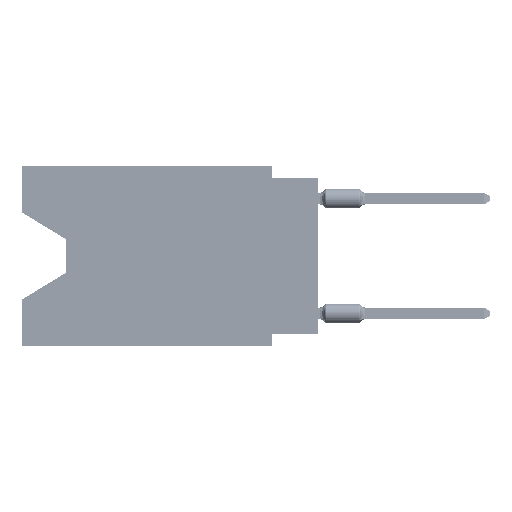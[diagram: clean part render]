
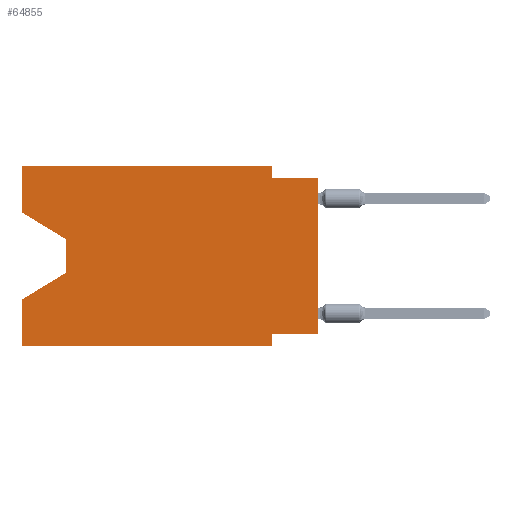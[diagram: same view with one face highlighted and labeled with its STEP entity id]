
A CAD part, left-side view. The second image highlights one B-rep face of the part: STEP entity #64855.
In plain terms, the highlighted planar face has unit normal (-1, 0, 0).
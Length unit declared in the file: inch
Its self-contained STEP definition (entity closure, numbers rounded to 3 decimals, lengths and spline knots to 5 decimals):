
#2189 = DIRECTION ( 'NONE',  ( 0., 0., -1. ) ) ;
#3252 = ORIENTED_EDGE ( 'NONE', *, *, #37040, .F. ) ;
#3545 = VERTEX_POINT ( 'NONE', #38048 ) ;
#3946 = LINE ( 'NONE', #55321, #9532 ) ;
#5629 = CARTESIAN_POINT ( 'NONE',  ( 0., 0.645, 0. ) ) ;
#6065 = ORIENTED_EDGE ( 'NONE', *, *, #27623, .T. ) ;
#6463 = EDGE_CURVE ( 'NONE', #42686, #31544, #49283, .T. ) ;
#7975 = VERTEX_POINT ( 'NONE', #44523 ) ;
#8594 = VERTEX_POINT ( 'NONE', #43351 ) ;
#9532 = VECTOR ( 'NONE', #60090, 39.37008 ) ;
#11187 = DIRECTION ( 'NONE',  ( 0., 0., -1. ) ) ;
#11610 = EDGE_CURVE ( 'NONE', #42686, #52033, #26875, .T. ) ;
#12078 = LINE ( 'NONE', #22346, #57967 ) ;
#12210 = VECTOR ( 'NONE', #60631, 39.37008 ) ;
#12718 = VERTEX_POINT ( 'NONE', #13309 ) ;
#12744 = LINE ( 'NONE', #13426, #60323 ) ;
#13309 = CARTESIAN_POINT ( 'NONE',  ( 0., 0.1, -0.39 ) ) ;
#13426 = CARTESIAN_POINT ( 'NONE',  ( 0., 0., 0. ) ) ;
#14960 = LINE ( 'NONE', #51950, #60369 ) ;
#16079 = ORIENTED_EDGE ( 'NONE', *, *, #6463, .F. ) ;
#16603 = CARTESIAN_POINT ( 'NONE',  ( 0., 0.645, -0.39 ) ) ;
#16934 = VECTOR ( 'NONE', #54395, 39.37008 ) ;
#17810 = CARTESIAN_POINT ( 'NONE',  ( 0., 0.645, -0.10025 ) ) ;
#17923 = FACE_OUTER_BOUND ( 'NONE', #52708, .T. ) ;
#19868 = CARTESIAN_POINT ( 'NONE',  ( 0., 0., -0.025 ) ) ;
#20145 = ORIENTED_EDGE ( 'NONE', *, *, #11610, .T. ) ;
#20229 = ORIENTED_EDGE ( 'NONE', *, *, #62414, .T. ) ;
#20621 = CARTESIAN_POINT ( 'NONE',  ( 0., 0.55, -0.158 ) ) ;
#20980 = CARTESIAN_POINT ( 'NONE',  ( 0., 0.645, -0.39 ) ) ;
#21755 = AXIS2_PLACEMENT_3D ( 'NONE', #59343, #28201, #2189 ) ;
#21877 = EDGE_CURVE ( 'NONE', #61639, #3545, #3946, .T. ) ;
#22346 = CARTESIAN_POINT ( 'NONE',  ( 0., 0.1, 0. ) ) ;
#22469 = VECTOR ( 'NONE', #64134, 39.37008 ) ;
#23143 = CARTESIAN_POINT ( 'NONE',  ( 0., 0.645, -0.28975 ) ) ;
#24936 = EDGE_CURVE ( 'NONE', #52033, #7975, #57927, .T. ) ;
#25849 = DIRECTION ( 'NONE',  ( 0., -0.855, -0.519 ) ) ;
#26875 = LINE ( 'NONE', #31321, #52584 ) ;
#27525 = ORIENTED_EDGE ( 'NONE', *, *, #64669, .F. ) ;
#27623 = EDGE_CURVE ( 'NONE', #7975, #59169, #54735, .T. ) ;
#28201 = DIRECTION ( 'NONE',  ( 1., 0., 0. ) ) ;
#28470 = ORIENTED_EDGE ( 'NONE', *, *, #21877, .F. ) ;
#28643 = ORIENTED_EDGE ( 'NONE', *, *, #33862, .F. ) ;
#29170 = DIRECTION ( 'NONE',  ( 0., 0., 1. ) ) ;
#30195 = EDGE_CURVE ( 'NONE', #53446, #51145, #45559, .T. ) ;
#30322 = VECTOR ( 'NONE', #57950, 39.37008 ) ;
#31321 = CARTESIAN_POINT ( 'NONE',  ( 0., 0.645, -0.10025 ) ) ;
#31506 = CARTESIAN_POINT ( 'NONE',  ( 0., 0., -0.025 ) ) ;
#31544 = VERTEX_POINT ( 'NONE', #57718 ) ;
#33500 = CARTESIAN_POINT ( 'NONE',  ( 0., 0.55, -0.232 ) ) ;
#33862 = EDGE_CURVE ( 'NONE', #3545, #12718, #14960, .T. ) ;
#34720 = CARTESIAN_POINT ( 'NONE',  ( 0., 0.1, -0.025 ) ) ;
#35931 = EDGE_CURVE ( 'NONE', #61639, #51145, #12744, .T. ) ;
#37040 = EDGE_CURVE ( 'NONE', #8594, #53446, #12078, .T. ) ;
#38048 = CARTESIAN_POINT ( 'NONE',  ( 0., 0.1, -0.365 ) ) ;
#38473 = PLANE ( 'NONE',  #21755 ) ;
#38944 = ORIENTED_EDGE ( 'NONE', *, *, #35931, .T. ) ;
#41933 = CARTESIAN_POINT ( 'NONE',  ( 0., 0.645, 0. ) ) ;
#42197 = DIRECTION ( 'NONE',  ( 0., 0., -1. ) ) ;
#42686 = VERTEX_POINT ( 'NONE', #17810 ) ;
#43008 = EDGE_CURVE ( 'NONE', #31544, #8594, #57991, .T. ) ;
#43351 = CARTESIAN_POINT ( 'NONE',  ( 0., 0.1, 0. ) ) ;
#44033 = ORIENTED_EDGE ( 'NONE', *, *, #24936, .T. ) ;
#44523 = CARTESIAN_POINT ( 'NONE',  ( 0., 0.55, -0.232 ) ) ;
#44737 = VECTOR ( 'NONE', #52885, 39.37008 ) ;
#45559 = LINE ( 'NONE', #19868, #12210 ) ;
#47347 = VECTOR ( 'NONE', #42197, 39.37008 ) ;
#48123 = ORIENTED_EDGE ( 'NONE', *, *, #30195, .F. ) ;
#48268 = CARTESIAN_POINT ( 'NONE',  ( 0., 0.645, 0. ) ) ;
#48484 = VERTEX_POINT ( 'NONE', #16603 ) ;
#49119 = CARTESIAN_POINT ( 'NONE',  ( 0., 0.55, -0.158 ) ) ;
#49283 = LINE ( 'NONE', #48268, #63773 ) ;
#49627 = DIRECTION ( 'NONE',  ( 0., 0., 1. ) ) ;
#51145 = VERTEX_POINT ( 'NONE', #31506 ) ;
#51950 = CARTESIAN_POINT ( 'NONE',  ( 0., 0.1, -0.39 ) ) ;
#52033 = VERTEX_POINT ( 'NONE', #49119 ) ;
#52584 = VECTOR ( 'NONE', #25849, 39.37008 ) ;
#52708 = EDGE_LOOP ( 'NONE', ( #20145, #44033, #6065, #27525, #20229, #28643, #28470, #38944, #48123, #3252, #52871, #16079 ) ) ;
#52871 = ORIENTED_EDGE ( 'NONE', *, *, #43008, .F. ) ;
#52885 = DIRECTION ( 'NONE',  ( 0., 0., 1. ) ) ;
#53079 = CARTESIAN_POINT ( 'NONE',  ( 0., 0., -0.365 ) ) ;
#53446 = VERTEX_POINT ( 'NONE', #34720 ) ;
#54395 = DIRECTION ( 'NONE',  ( 0., 0.855, -0.519 ) ) ;
#54735 = LINE ( 'NONE', #33500, #16934 ) ;
#55321 = CARTESIAN_POINT ( 'NONE',  ( 0., 0., -0.365 ) ) ;
#57718 = CARTESIAN_POINT ( 'NONE',  ( 0., 0.645, 0. ) ) ;
#57927 = LINE ( 'NONE', #20621, #47347 ) ;
#57950 = DIRECTION ( 'NONE',  ( 0., -1., 0. ) ) ;
#57967 = VECTOR ( 'NONE', #58629, 39.37008 ) ;
#57991 = LINE ( 'NONE', #5629, #22469 ) ;
#58629 = DIRECTION ( 'NONE',  ( 0., 0., -1. ) ) ;
#59169 = VERTEX_POINT ( 'NONE', #23143 ) ;
#59343 = CARTESIAN_POINT ( 'NONE',  ( 0., 0.645, 0. ) ) ;
#60090 = DIRECTION ( 'NONE',  ( 0., 1., 0. ) ) ;
#60323 = VECTOR ( 'NONE', #29170, 39.37008 ) ;
#60369 = VECTOR ( 'NONE', #11187, 39.37008 ) ;
#60631 = DIRECTION ( 'NONE',  ( 0., -1., 0. ) ) ;
#61639 = VERTEX_POINT ( 'NONE', #53079 ) ;
#62414 = EDGE_CURVE ( 'NONE', #48484, #12718, #63079, .T. ) ;
#63079 = LINE ( 'NONE', #20980, #30322 ) ;
#63131 = LINE ( 'NONE', #41933, #44737 ) ;
#63773 = VECTOR ( 'NONE', #49627, 39.37008 ) ;
#64134 = DIRECTION ( 'NONE',  ( 0., -1., 0. ) ) ;
#64669 = EDGE_CURVE ( 'NONE', #48484, #59169, #63131, .T. ) ;
#64855 = ADVANCED_FACE ( 'NONE', ( #17923 ), #38473, .F. ) ;
